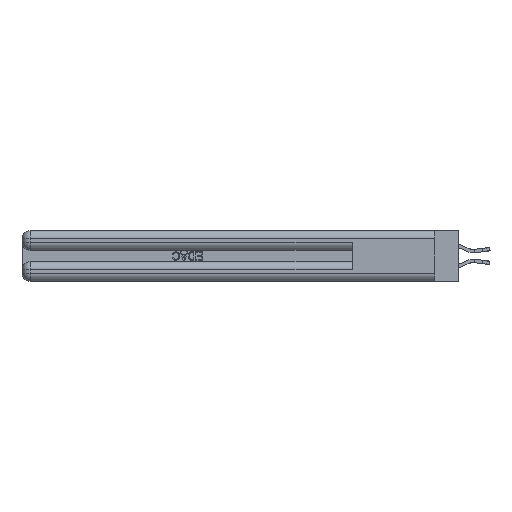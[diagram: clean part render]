
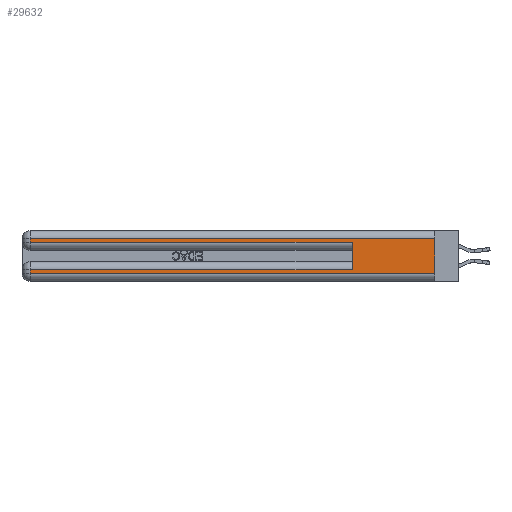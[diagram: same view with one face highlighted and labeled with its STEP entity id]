
A CAD part, left-side view. The second image highlights one B-rep face of the part: STEP entity #29632.
In plain terms, the highlighted planar face has unit normal (-1, 0, 0).
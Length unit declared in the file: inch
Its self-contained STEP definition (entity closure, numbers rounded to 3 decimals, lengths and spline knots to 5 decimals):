
#998 = EDGE_LOOP ( 'NONE', ( #24378, #38094, #37293, #13509, #18380, #32396, #26389, #2138 ) ) ;
#1020 = VECTOR ( 'NONE', #7317, 39.37008 ) ;
#1661 = LINE ( 'NONE', #27306, #33508 ) ;
#2138 = ORIENTED_EDGE ( 'NONE', *, *, #29311, .T. ) ;
#3830 = VERTEX_POINT ( 'NONE', #16865 ) ;
#4081 = DIRECTION ( 'NONE',  ( 1., 0., 0. ) ) ;
#5679 = EDGE_CURVE ( 'NONE', #36717, #3830, #36226, .T. ) ;
#7317 = DIRECTION ( 'NONE',  ( 0., 0., -1. ) ) ;
#8569 = DIRECTION ( 'NONE',  ( 0., 1., 0. ) ) ;
#9123 = CARTESIAN_POINT ( 'NONE',  ( 0., 0., 0.06 ) ) ;
#9559 = LINE ( 'NONE', #37014, #26924 ) ;
#10338 = VERTEX_POINT ( 'NONE', #39743 ) ;
#10965 = EDGE_CURVE ( 'NONE', #10338, #31332, #28676, .T. ) ;
#11560 = LINE ( 'NONE', #9123, #37594 ) ;
#12129 = CARTESIAN_POINT ( 'NONE',  ( 0., 0., 0.31 ) ) ;
#13428 = VECTOR ( 'NONE', #17467, 39.37008 ) ;
#13509 = ORIENTED_EDGE ( 'NONE', *, *, #24180, .T. ) ;
#13690 = VECTOR ( 'NONE', #8569, 39.37008 ) ;
#14612 = EDGE_CURVE ( 'NONE', #10338, #18442, #20680, .T. ) ;
#14716 = DIRECTION ( 'NONE',  ( 0., 0., -1. ) ) ;
#16047 = VERTEX_POINT ( 'NONE', #38252 ) ;
#16865 = CARTESIAN_POINT ( 'NONE',  ( 0., 0., 0.06 ) ) ;
#17236 = LINE ( 'NONE', #21828, #24481 ) ;
#17332 = CARTESIAN_POINT ( 'NONE',  ( 0., 0.6, 0.145 ) ) ;
#17467 = DIRECTION ( 'NONE',  ( 0., 0., 1. ) ) ;
#17880 = VERTEX_POINT ( 'NONE', #28031 ) ;
#17996 = DIRECTION ( 'NONE',  ( 0., 1., 0. ) ) ;
#18273 = LINE ( 'NONE', #33179, #20663 ) ;
#18380 = ORIENTED_EDGE ( 'NONE', *, *, #14612, .F. ) ;
#18442 = VERTEX_POINT ( 'NONE', #25155 ) ;
#18693 = DIRECTION ( 'NONE',  ( 0., 0., -1. ) ) ;
#19865 = VERTEX_POINT ( 'NONE', #39463 ) ;
#19905 = AXIS2_PLACEMENT_3D ( 'NONE', #28514, #4081, #31610 ) ;
#20663 = VECTOR ( 'NONE', #14716, 39.37008 ) ;
#20680 = LINE ( 'NONE', #17332, #13428 ) ;
#21828 = CARTESIAN_POINT ( 'NONE',  ( 0., 0., 0.285 ) ) ;
#22648 = FACE_OUTER_BOUND ( 'NONE', #998, .T. ) ;
#24180 = EDGE_CURVE ( 'NONE', #19865, #18442, #17236, .T. ) ;
#24378 = ORIENTED_EDGE ( 'NONE', *, *, #5679, .F. ) ;
#24481 = VECTOR ( 'NONE', #28012, 39.37008 ) ;
#25155 = CARTESIAN_POINT ( 'NONE',  ( 0., 0.6, 0.285 ) ) ;
#25652 = CARTESIAN_POINT ( 'NONE',  ( 0., 0., 0.37 ) ) ;
#26389 = ORIENTED_EDGE ( 'NONE', *, *, #35583, .T. ) ;
#26924 = VECTOR ( 'NONE', #18693, 39.37008 ) ;
#27306 = CARTESIAN_POINT ( 'NONE',  ( 0., 0., 0.31 ) ) ;
#28012 = DIRECTION ( 'NONE',  ( 0., -1., 0. ) ) ;
#28031 = CARTESIAN_POINT ( 'NONE',  ( 0., 2.94, 0.06 ) ) ;
#28514 = CARTESIAN_POINT ( 'NONE',  ( 0., 0., 0.37 ) ) ;
#28676 = LINE ( 'NONE', #36464, #13690 ) ;
#29311 = EDGE_CURVE ( 'NONE', #17880, #3830, #11560, .T. ) ;
#29632 = ADVANCED_FACE ( 'NONE', ( #22648 ), #32021, .F. ) ;
#30017 = EDGE_CURVE ( 'NONE', #16047, #19865, #18273, .T. ) ;
#31027 = EDGE_CURVE ( 'NONE', #36717, #16047, #1661, .T. ) ;
#31332 = VERTEX_POINT ( 'NONE', #38027 ) ;
#31610 = DIRECTION ( 'NONE',  ( 0., 0., -1. ) ) ;
#32021 = PLANE ( 'NONE',  #19905 ) ;
#32396 = ORIENTED_EDGE ( 'NONE', *, *, #10965, .T. ) ;
#33179 = CARTESIAN_POINT ( 'NONE',  ( 0., 2.94, 0.37 ) ) ;
#33369 = DIRECTION ( 'NONE',  ( 0., -1., 0. ) ) ;
#33508 = VECTOR ( 'NONE', #17996, 39.37008 ) ;
#35583 = EDGE_CURVE ( 'NONE', #31332, #17880, #9559, .T. ) ;
#36226 = LINE ( 'NONE', #25652, #1020 ) ;
#36464 = CARTESIAN_POINT ( 'NONE',  ( 0., 0., 0.085 ) ) ;
#36717 = VERTEX_POINT ( 'NONE', #12129 ) ;
#37014 = CARTESIAN_POINT ( 'NONE',  ( 0., 2.94, 0.37 ) ) ;
#37293 = ORIENTED_EDGE ( 'NONE', *, *, #30017, .T. ) ;
#37594 = VECTOR ( 'NONE', #33369, 39.37008 ) ;
#38027 = CARTESIAN_POINT ( 'NONE',  ( 0., 2.94, 0.085 ) ) ;
#38094 = ORIENTED_EDGE ( 'NONE', *, *, #31027, .T. ) ;
#38252 = CARTESIAN_POINT ( 'NONE',  ( 0., 2.94, 0.31 ) ) ;
#39463 = CARTESIAN_POINT ( 'NONE',  ( 0., 2.94, 0.285 ) ) ;
#39743 = CARTESIAN_POINT ( 'NONE',  ( 0., 0.6, 0.085 ) ) ;
